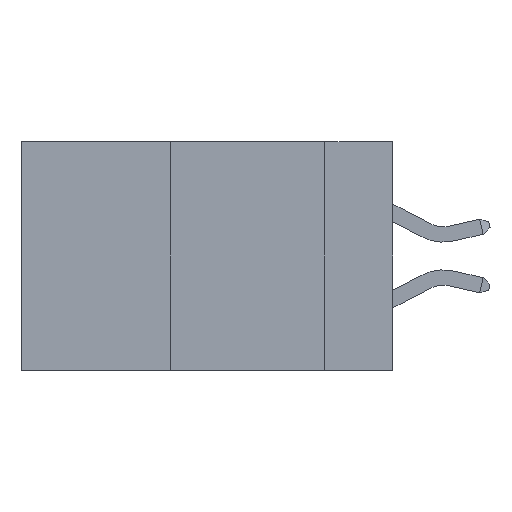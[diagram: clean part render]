
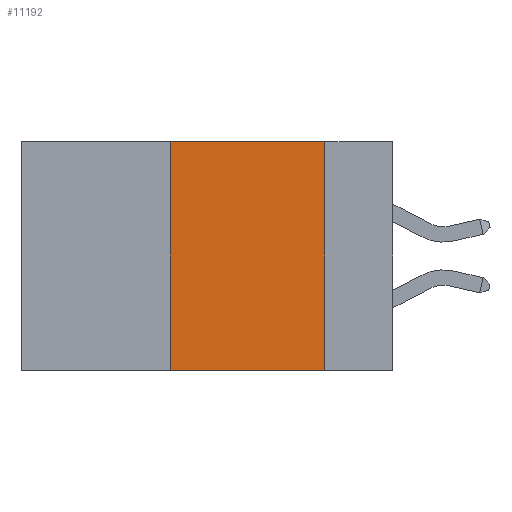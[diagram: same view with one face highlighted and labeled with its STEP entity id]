
A CAD part, left-side view. The second image highlights one B-rep face of the part: STEP entity #11192.
In plain terms, the highlighted planar face has unit normal (-1, 0, 0).
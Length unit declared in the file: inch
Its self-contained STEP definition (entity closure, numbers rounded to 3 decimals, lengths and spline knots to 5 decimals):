
#285 = FACE_OUTER_BOUND ( 'NONE', #1312, .T. ) ;
#862 = ORIENTED_EDGE ( 'NONE', *, *, #11500, .F. ) ;
#992 = VERTEX_POINT ( 'NONE', #3485 ) ;
#1312 = EDGE_LOOP ( 'NONE', ( #862, #4873, #10647, #7926 ) ) ;
#1447 = CARTESIAN_POINT ( 'NONE',  ( 0., 0.11, 0. ) ) ;
#1921 = CARTESIAN_POINT ( 'NONE',  ( 0., 0.6, 0. ) ) ;
#2149 = DIRECTION ( 'NONE',  ( 1., 0., 0. ) ) ;
#2325 = VERTEX_POINT ( 'NONE', #4747 ) ;
#2355 = VECTOR ( 'NONE', #9386, 39.37008 ) ;
#2624 = EDGE_CURVE ( 'NONE', #992, #11935, #3362, .T. ) ;
#2896 = DIRECTION ( 'NONE',  ( 0., 0., -1. ) ) ;
#3362 = LINE ( 'NONE', #7152, #6829 ) ;
#3485 = CARTESIAN_POINT ( 'NONE',  ( 0., 0.36, -0.37 ) ) ;
#3980 = AXIS2_PLACEMENT_3D ( 'NONE', #10669, #2149, #2896 ) ;
#4300 = CARTESIAN_POINT ( 'NONE',  ( 0., 0.11, -0.37 ) ) ;
#4747 = CARTESIAN_POINT ( 'NONE',  ( 0., 0.36, 0. ) ) ;
#4873 = ORIENTED_EDGE ( 'NONE', *, *, #9684, .F. ) ;
#4990 = VECTOR ( 'NONE', #10842, 39.37008 ) ;
#6408 = LINE ( 'NONE', #10089, #8882 ) ;
#6829 = VECTOR ( 'NONE', #8026, 39.37008 ) ;
#7152 = CARTESIAN_POINT ( 'NONE',  ( 0., 0.6, -0.37 ) ) ;
#7208 = DIRECTION ( 'NONE',  ( 0., 0., 1. ) ) ;
#7926 = ORIENTED_EDGE ( 'NONE', *, *, #2624, .T. ) ;
#8026 = DIRECTION ( 'NONE',  ( 0., -1., 0. ) ) ;
#8114 = VERTEX_POINT ( 'NONE', #8148 ) ;
#8148 = CARTESIAN_POINT ( 'NONE',  ( 0., 0.11, 0. ) ) ;
#8159 = EDGE_CURVE ( 'NONE', #992, #2325, #6408, .T. ) ;
#8882 = VECTOR ( 'NONE', #7208, 39.37008 ) ;
#9386 = DIRECTION ( 'NONE',  ( 0., -1., 0. ) ) ;
#9684 = EDGE_CURVE ( 'NONE', #2325, #8114, #11545, .T. ) ;
#9789 = LINE ( 'NONE', #1447, #4990 ) ;
#10089 = CARTESIAN_POINT ( 'NONE',  ( 0., 0.36, 0. ) ) ;
#10647 = ORIENTED_EDGE ( 'NONE', *, *, #8159, .F. ) ;
#10669 = CARTESIAN_POINT ( 'NONE',  ( 0., 0.6, 0. ) ) ;
#10842 = DIRECTION ( 'NONE',  ( 0., 0., -1. ) ) ;
#11192 = ADVANCED_FACE ( 'NONE', ( #285 ), #11404, .F. ) ;
#11404 = PLANE ( 'NONE',  #3980 ) ;
#11500 = EDGE_CURVE ( 'NONE', #8114, #11935, #9789, .T. ) ;
#11545 = LINE ( 'NONE', #1921, #2355 ) ;
#11935 = VERTEX_POINT ( 'NONE', #4300 ) ;
